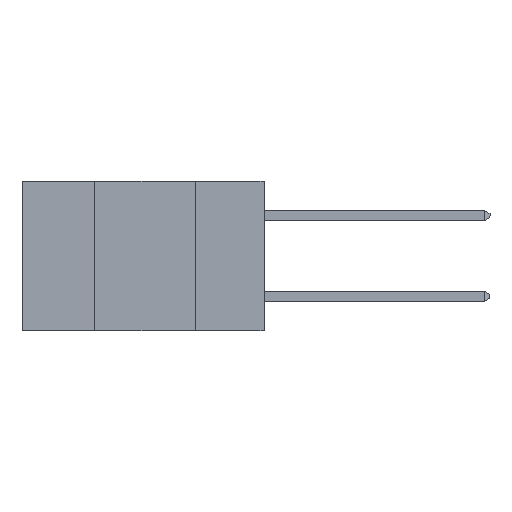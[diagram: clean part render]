
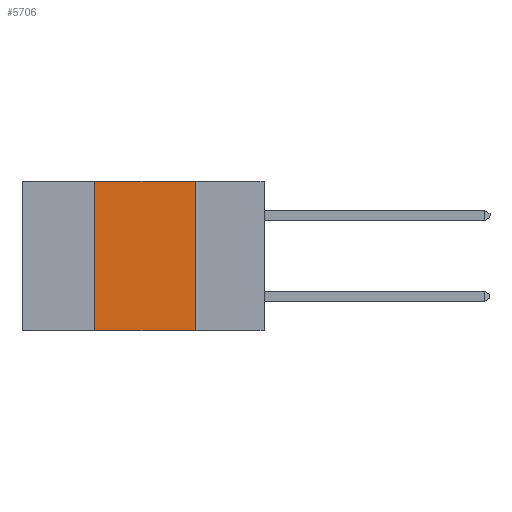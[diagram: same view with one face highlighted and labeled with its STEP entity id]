
A CAD part, left-side view. The second image highlights one B-rep face of the part: STEP entity #5706.
In plain terms, the highlighted planar face has unit normal (-1, 0, 0).
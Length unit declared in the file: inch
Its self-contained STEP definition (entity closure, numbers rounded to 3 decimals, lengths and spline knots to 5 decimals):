
#639 = DIRECTION ( 'NONE',  ( 0., 0., -1. ) ) ;
#1919 = DIRECTION ( 'NONE',  ( 1., 0., 0. ) ) ;
#2437 = DIRECTION ( 'NONE',  ( 0., 0., 1. ) ) ;
#2530 = VECTOR ( 'NONE', #15662, 39.37008 ) ;
#3258 = CARTESIAN_POINT ( 'NONE',  ( 0., 0.6, 0. ) ) ;
#5571 = FACE_OUTER_BOUND ( 'NONE', #21879, .T. ) ;
#5706 = ADVANCED_FACE ( 'NONE', ( #5571 ), #5791, .F. ) ;
#5785 = AXIS2_PLACEMENT_3D ( 'NONE', #3258, #1919, #639 ) ;
#5791 = PLANE ( 'NONE',  #5785 ) ;
#6154 = ORIENTED_EDGE ( 'NONE', *, *, #10710, .T. ) ;
#6375 = LINE ( 'NONE', #18462, #20614 ) ;
#6501 = VECTOR ( 'NONE', #20397, 39.37008 ) ;
#7927 = CARTESIAN_POINT ( 'NONE',  ( 0., 0.6, -0.37 ) ) ;
#8444 = CARTESIAN_POINT ( 'NONE',  ( 0., 0.17, 0. ) ) ;
#9037 = VERTEX_POINT ( 'NONE', #10964 ) ;
#9944 = ORIENTED_EDGE ( 'NONE', *, *, #12795, .F. ) ;
#10111 = VERTEX_POINT ( 'NONE', #11742 ) ;
#10354 = DIRECTION ( 'NONE',  ( 0., -1., 0. ) ) ;
#10710 = EDGE_CURVE ( 'NONE', #10111, #14972, #10766, .T. ) ;
#10766 = LINE ( 'NONE', #7927, #6501 ) ;
#10964 = CARTESIAN_POINT ( 'NONE',  ( 0., 0.17, 0. ) ) ;
#11419 = ORIENTED_EDGE ( 'NONE', *, *, #18139, .F. ) ;
#11742 = CARTESIAN_POINT ( 'NONE',  ( 0., 0.42, -0.37 ) ) ;
#12795 = EDGE_CURVE ( 'NONE', #10111, #21703, #6375, .T. ) ;
#14444 = VECTOR ( 'NONE', #10354, 39.37008 ) ;
#14972 = VERTEX_POINT ( 'NONE', #22551 ) ;
#14995 = LINE ( 'NONE', #15663, #14444 ) ;
#15662 = DIRECTION ( 'NONE',  ( 0., 0., -1. ) ) ;
#15663 = CARTESIAN_POINT ( 'NONE',  ( 0., 0.6, 0. ) ) ;
#15964 = CARTESIAN_POINT ( 'NONE',  ( 0., 0.42, 0. ) ) ;
#18139 = EDGE_CURVE ( 'NONE', #21703, #9037, #14995, .T. ) ;
#18462 = CARTESIAN_POINT ( 'NONE',  ( 0., 0.42, 0. ) ) ;
#20397 = DIRECTION ( 'NONE',  ( 0., -1., 0. ) ) ;
#20614 = VECTOR ( 'NONE', #2437, 39.37008 ) ;
#20831 = ORIENTED_EDGE ( 'NONE', *, *, #21428, .F. ) ;
#21428 = EDGE_CURVE ( 'NONE', #9037, #14972, #21475, .T. ) ;
#21475 = LINE ( 'NONE', #8444, #2530 ) ;
#21703 = VERTEX_POINT ( 'NONE', #15964 ) ;
#21879 = EDGE_LOOP ( 'NONE', ( #20831, #11419, #9944, #6154 ) ) ;
#22551 = CARTESIAN_POINT ( 'NONE',  ( 0., 0.17, -0.37 ) ) ;
